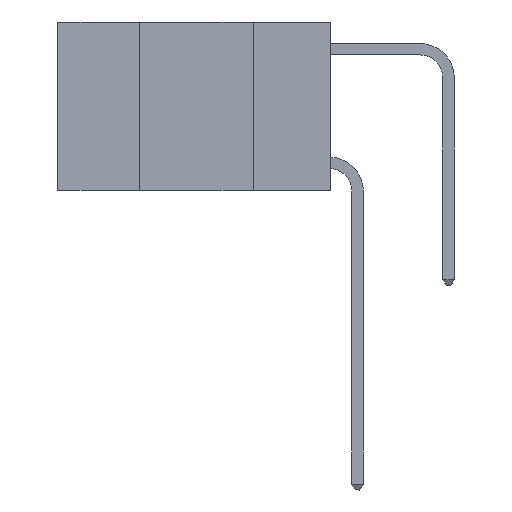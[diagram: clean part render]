
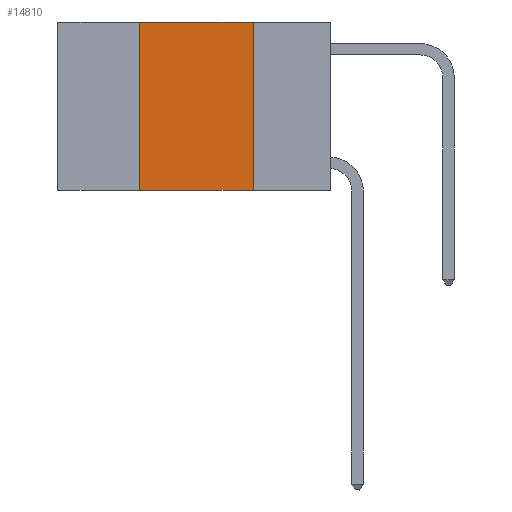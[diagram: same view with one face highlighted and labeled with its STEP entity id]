
A CAD part, left-side view. The second image highlights one B-rep face of the part: STEP entity #14810.
In plain terms, the highlighted planar face has unit normal (-1, 0, 0).
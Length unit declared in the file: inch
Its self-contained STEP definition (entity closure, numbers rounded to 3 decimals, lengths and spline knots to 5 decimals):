
#379 = EDGE_CURVE ( 'NONE', #11841, #7608, #10834, .T. ) ;
#1450 = CARTESIAN_POINT ( 'NONE',  ( 0., 0.17, 0. ) ) ;
#3183 = EDGE_CURVE ( 'NONE', #7608, #13991, #14327, .T. ) ;
#3466 = VECTOR ( 'NONE', #17691, 39.37008 ) ;
#4003 = EDGE_CURVE ( 'NONE', #11841, #17910, #9099, .T. ) ;
#4046 = EDGE_LOOP ( 'NONE', ( #16398, #13990, #14423, #4704 ) ) ;
#4113 = CARTESIAN_POINT ( 'NONE',  ( 0., 0.17, -0.37 ) ) ;
#4402 = VECTOR ( 'NONE', #8381, 39.37008 ) ;
#4443 = CARTESIAN_POINT ( 'NONE',  ( 0., 0.17, 0. ) ) ;
#4699 = FACE_OUTER_BOUND ( 'NONE', #4046, .T. ) ;
#4704 = ORIENTED_EDGE ( 'NONE', *, *, #4003, .T. ) ;
#4822 = LINE ( 'NONE', #1450, #4402 ) ;
#6212 = PLANE ( 'NONE',  #12823 ) ;
#7586 = DIRECTION ( 'NONE',  ( 0., 0., -1. ) ) ;
#7608 = VERTEX_POINT ( 'NONE', #15242 ) ;
#8381 = DIRECTION ( 'NONE',  ( 0., 0., -1. ) ) ;
#8681 = VECTOR ( 'NONE', #13134, 39.37008 ) ;
#9099 = LINE ( 'NONE', #17290, #8681 ) ;
#10026 = CARTESIAN_POINT ( 'NONE',  ( 0., 0.6, 0. ) ) ;
#10644 = VECTOR ( 'NONE', #14202, 39.37008 ) ;
#10834 = LINE ( 'NONE', #13205, #3466 ) ;
#11662 = CARTESIAN_POINT ( 'NONE',  ( 0., 0.6, 0. ) ) ;
#11841 = VERTEX_POINT ( 'NONE', #16305 ) ;
#12823 = AXIS2_PLACEMENT_3D ( 'NONE', #11662, #15865, #7586 ) ;
#13134 = DIRECTION ( 'NONE',  ( 0., -1., 0. ) ) ;
#13205 = CARTESIAN_POINT ( 'NONE',  ( 0., 0.42, 0. ) ) ;
#13990 = ORIENTED_EDGE ( 'NONE', *, *, #3183, .F. ) ;
#13991 = VERTEX_POINT ( 'NONE', #4443 ) ;
#14202 = DIRECTION ( 'NONE',  ( 0., -1., 0. ) ) ;
#14327 = LINE ( 'NONE', #10026, #10644 ) ;
#14423 = ORIENTED_EDGE ( 'NONE', *, *, #379, .F. ) ;
#14810 = ADVANCED_FACE ( 'NONE', ( #4699 ), #6212, .F. ) ;
#15242 = CARTESIAN_POINT ( 'NONE',  ( 0., 0.42, 0. ) ) ;
#15865 = DIRECTION ( 'NONE',  ( 1., 0., 0. ) ) ;
#16305 = CARTESIAN_POINT ( 'NONE',  ( 0., 0.42, -0.37 ) ) ;
#16398 = ORIENTED_EDGE ( 'NONE', *, *, #16422, .F. ) ;
#16422 = EDGE_CURVE ( 'NONE', #13991, #17910, #4822, .T. ) ;
#17290 = CARTESIAN_POINT ( 'NONE',  ( 0., 0.6, -0.37 ) ) ;
#17691 = DIRECTION ( 'NONE',  ( 0., 0., 1. ) ) ;
#17910 = VERTEX_POINT ( 'NONE', #4113 ) ;
